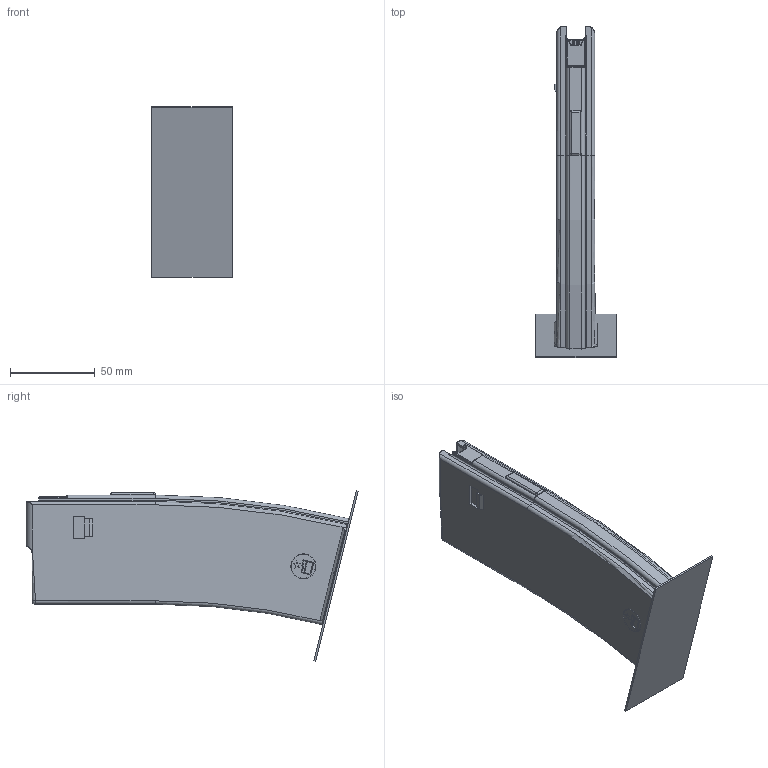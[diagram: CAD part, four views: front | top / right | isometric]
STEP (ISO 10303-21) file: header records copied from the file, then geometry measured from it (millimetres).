
FILE_DESCRIPTION(/* description */ ('STEP AP214'),/* implementation_level */ '2;1');
FILE_NAME(/* name */ 'Ivan''Ivan''s Standard Mag Body.stp',/* time_stamp */ '2019-01-27T20:55:40-06:00',/* author */ ('johne'),/* organization */ (''),/* preprocessor_version */ 'ST-DEVELOPER v16.13',/* originating_system */ 'Autodesk Inventor 2018',/* authorisation */ '');
FILE_SCHEMA (('AUTOMOTIVE_DESIGN { 1 0 10303 214 3 1 1 }'));
Length unit declared in the file: millimetre
Products named in the file (1): doodoo
Bounding box: 47.67 x 196.24 x 100.95 mm (x, y, z)
Volume: 77784.2 mm3; surface area: 70087.1 mm2
Topology: 7 solids, 7 shells, 481 faces, 1229 edges, 748 vertices
Faces by surface type: plane 171, cylinder 152, bspline 97, torus 51, sphere 6, cone 4
Full cylindrical faces by diameter (mm): 14.072 x2
Entity records: 24586 total; most frequent: CARTESIAN_POINT 13493, ORIENTED_EDGE 2414, DIRECTION 2187, EDGE_CURVE 1207, AXIS2_PLACEMENT_3D 801, VERTEX_POINT 746, LINE 585, VECTOR 585
